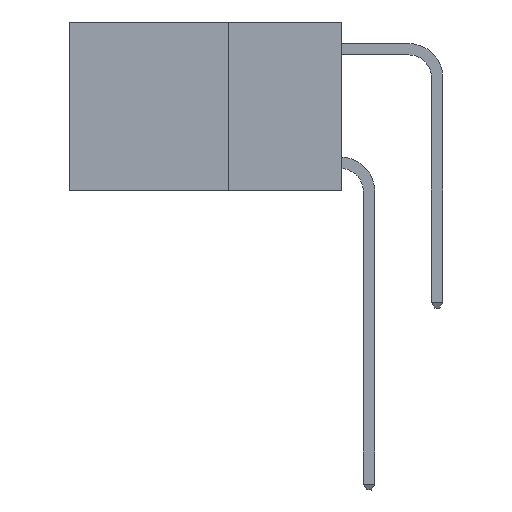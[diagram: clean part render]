
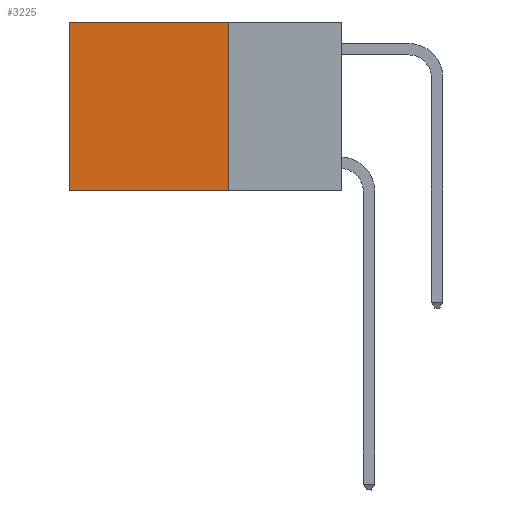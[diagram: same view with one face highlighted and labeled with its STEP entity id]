
A CAD part, left-side view. The second image highlights one B-rep face of the part: STEP entity #3225.
In plain terms, the highlighted planar face has unit normal (-1, 0, 0).
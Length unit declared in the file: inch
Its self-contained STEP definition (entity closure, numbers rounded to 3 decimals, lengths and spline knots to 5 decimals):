
#159 = LINE ( 'NONE', #14268, #3016 ) ;
#1481 = VECTOR ( 'NONE', #16737, 39.37008 ) ;
#2236 = CARTESIAN_POINT ( 'NONE',  ( 0.2625, 0.25, -0.37 ) ) ;
#2282 = CARTESIAN_POINT ( 'NONE',  ( 0.2625, 0.6, -0.37 ) ) ;
#2887 = EDGE_LOOP ( 'NONE', ( #6765, #4711, #19481, #4425 ) ) ;
#3016 = VECTOR ( 'NONE', #11306, 39.37008 ) ;
#3225 = ADVANCED_FACE ( 'NONE', ( #9650 ), #9536, .F. ) ;
#3483 = VERTEX_POINT ( 'NONE', #7632 ) ;
#4425 = ORIENTED_EDGE ( 'NONE', *, *, #18527, .T. ) ;
#4711 = ORIENTED_EDGE ( 'NONE', *, *, #12929, .F. ) ;
#5479 = EDGE_CURVE ( 'NONE', #3483, #8860, #19194, .T. ) ;
#5980 = LINE ( 'NONE', #7322, #1481 ) ;
#6712 = AXIS2_PLACEMENT_3D ( 'NONE', #10974, #13849, #7820 ) ;
#6765 = ORIENTED_EDGE ( 'NONE', *, *, #5479, .T. ) ;
#7322 = CARTESIAN_POINT ( 'NONE',  ( 0.2625, 0.25, 0. ) ) ;
#7632 = CARTESIAN_POINT ( 'NONE',  ( 0.2625, 0.6, 0. ) ) ;
#7820 = DIRECTION ( 'NONE',  ( 0., 0., -1. ) ) ;
#8417 = VECTOR ( 'NONE', #16903, 39.37008 ) ;
#8860 = VERTEX_POINT ( 'NONE', #2282 ) ;
#9410 = CARTESIAN_POINT ( 'NONE',  ( 0.2625, 0.25, 0. ) ) ;
#9536 = PLANE ( 'NONE',  #6712 ) ;
#9650 = FACE_OUTER_BOUND ( 'NONE', #2887, .T. ) ;
#10118 = VECTOR ( 'NONE', #12786, 39.37008 ) ;
#10851 = CARTESIAN_POINT ( 'NONE',  ( 0.2625, 0.25, -0.37 ) ) ;
#10974 = CARTESIAN_POINT ( 'NONE',  ( 0.2625, 0.25, 0. ) ) ;
#11306 = DIRECTION ( 'NONE',  ( 0., 0., -1. ) ) ;
#12786 = DIRECTION ( 'NONE',  ( 0., 1., 0. ) ) ;
#12922 = EDGE_CURVE ( 'NONE', #18087, #13355, #159, .T. ) ;
#12929 = EDGE_CURVE ( 'NONE', #13355, #8860, #16001, .T. ) ;
#13355 = VERTEX_POINT ( 'NONE', #10851 ) ;
#13849 = DIRECTION ( 'NONE',  ( 1., 0., 0. ) ) ;
#13942 = CARTESIAN_POINT ( 'NONE',  ( 0.2625, 0.6, 0. ) ) ;
#14268 = CARTESIAN_POINT ( 'NONE',  ( 0.2625, 0.25, 0. ) ) ;
#16001 = LINE ( 'NONE', #2236, #10118 ) ;
#16737 = DIRECTION ( 'NONE',  ( 0., 1., 0. ) ) ;
#16903 = DIRECTION ( 'NONE',  ( 0., 0., -1. ) ) ;
#18087 = VERTEX_POINT ( 'NONE', #9410 ) ;
#18527 = EDGE_CURVE ( 'NONE', #18087, #3483, #5980, .T. ) ;
#19194 = LINE ( 'NONE', #13942, #8417 ) ;
#19481 = ORIENTED_EDGE ( 'NONE', *, *, #12922, .F. ) ;
